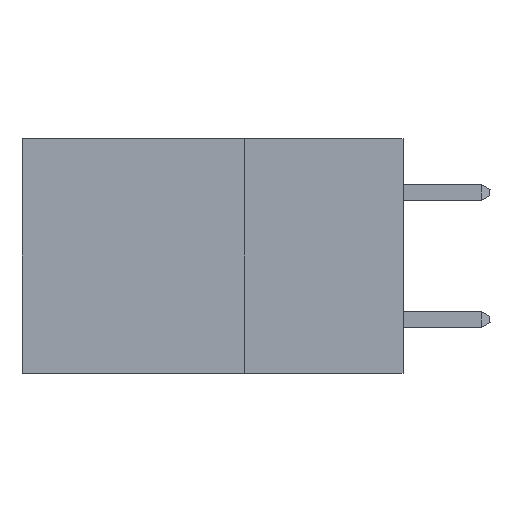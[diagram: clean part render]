
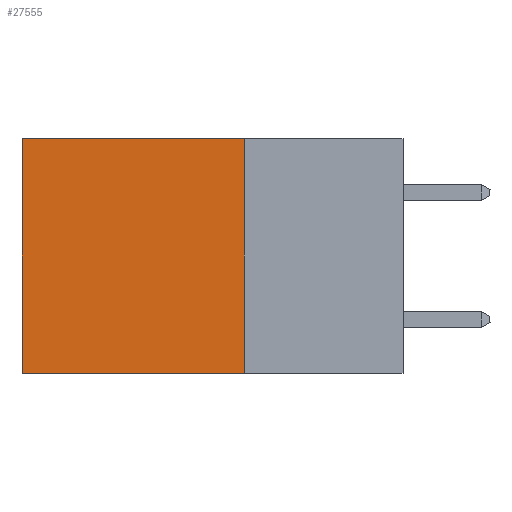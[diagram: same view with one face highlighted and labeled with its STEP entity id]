
A CAD part, left-side view. The second image highlights one B-rep face of the part: STEP entity #27555.
In plain terms, the highlighted planar face has unit normal (-1, 0, 0).
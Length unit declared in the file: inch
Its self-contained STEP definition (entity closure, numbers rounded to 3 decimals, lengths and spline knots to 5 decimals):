
#207 = VECTOR ( 'NONE', #13195, 39.37008 ) ;
#388 = ORIENTED_EDGE ( 'NONE', *, *, #19582, .F. ) ;
#765 = LINE ( 'NONE', #6176, #24434 ) ;
#1221 = CARTESIAN_POINT ( 'NONE',  ( 0.2875, 0.25, 0. ) ) ;
#1945 = AXIS2_PLACEMENT_3D ( 'NONE', #4879, #26766, #27080 ) ;
#1976 = VERTEX_POINT ( 'NONE', #7073 ) ;
#3349 = CARTESIAN_POINT ( 'NONE',  ( 0.2875, 0.6, -0.37 ) ) ;
#3914 = DIRECTION ( 'NONE',  ( 0., 0., -1. ) ) ;
#4311 = EDGE_CURVE ( 'NONE', #1976, #6995, #11002, .T. ) ;
#4879 = CARTESIAN_POINT ( 'NONE',  ( 0.2875, 0.25, 0. ) ) ;
#5512 = CARTESIAN_POINT ( 'NONE',  ( 0.2875, 0.6, 0. ) ) ;
#6122 = VERTEX_POINT ( 'NONE', #29059 ) ;
#6176 = CARTESIAN_POINT ( 'NONE',  ( 0.2875, 0.25, 0. ) ) ;
#6995 = VERTEX_POINT ( 'NONE', #5512 ) ;
#7073 = CARTESIAN_POINT ( 'NONE',  ( 0.2875, 0.25, 0. ) ) ;
#8618 = DIRECTION ( 'NONE',  ( 0., 1., 0. ) ) ;
#9057 = LINE ( 'NONE', #30421, #207 ) ;
#10440 = LINE ( 'NONE', #23267, #26053 ) ;
#10877 = EDGE_CURVE ( 'NONE', #6995, #17458, #9057, .T. ) ;
#11002 = LINE ( 'NONE', #1221, #17862 ) ;
#11140 = DIRECTION ( 'NONE',  ( 0., 1., 0. ) ) ;
#13195 = DIRECTION ( 'NONE',  ( 0., 0., -1. ) ) ;
#13988 = ORIENTED_EDGE ( 'NONE', *, *, #21840, .F. ) ;
#14839 = ORIENTED_EDGE ( 'NONE', *, *, #4311, .T. ) ;
#17458 = VERTEX_POINT ( 'NONE', #3349 ) ;
#17862 = VECTOR ( 'NONE', #8618, 39.37008 ) ;
#19483 = PLANE ( 'NONE',  #1945 ) ;
#19582 = EDGE_CURVE ( 'NONE', #6122, #17458, #10440, .T. ) ;
#21840 = EDGE_CURVE ( 'NONE', #1976, #6122, #765, .T. ) ;
#23267 = CARTESIAN_POINT ( 'NONE',  ( 0.2875, 0.25, -0.37 ) ) ;
#24434 = VECTOR ( 'NONE', #3914, 39.37008 ) ;
#25345 = EDGE_LOOP ( 'NONE', ( #30286, #388, #13988, #14839 ) ) ;
#26053 = VECTOR ( 'NONE', #11140, 39.37008 ) ;
#26766 = DIRECTION ( 'NONE',  ( 1., 0., 0. ) ) ;
#27016 = FACE_OUTER_BOUND ( 'NONE', #25345, .T. ) ;
#27080 = DIRECTION ( 'NONE',  ( 0., 0., -1. ) ) ;
#27555 = ADVANCED_FACE ( 'NONE', ( #27016 ), #19483, .F. ) ;
#29059 = CARTESIAN_POINT ( 'NONE',  ( 0.2875, 0.25, -0.37 ) ) ;
#30286 = ORIENTED_EDGE ( 'NONE', *, *, #10877, .T. ) ;
#30421 = CARTESIAN_POINT ( 'NONE',  ( 0.2875, 0.6, 0. ) ) ;
